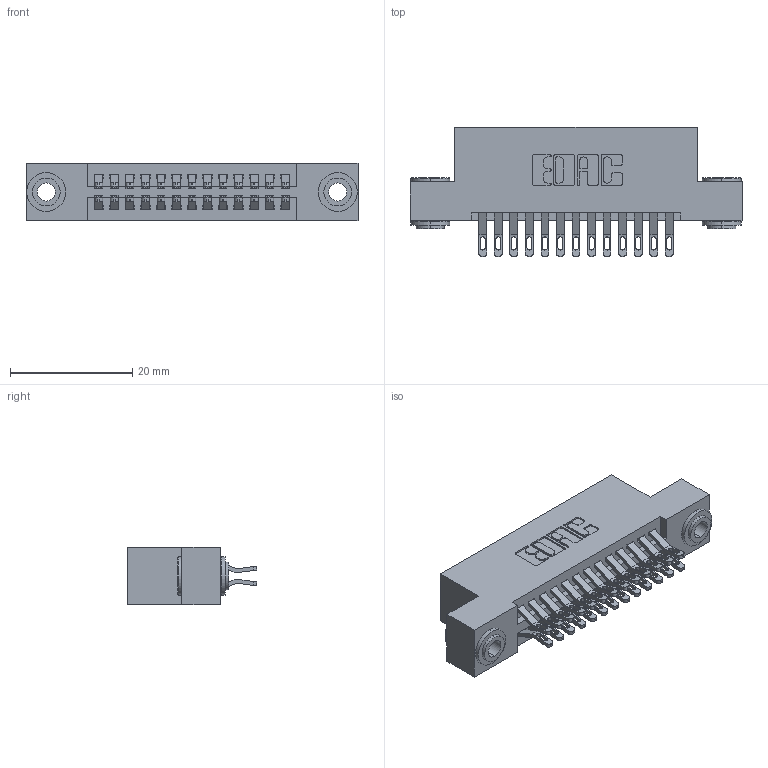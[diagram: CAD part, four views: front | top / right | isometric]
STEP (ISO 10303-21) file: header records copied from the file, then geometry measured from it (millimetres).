
FILE_DESCRIPTION (( 'STEP AP203' ), '1' );
FILE_NAME ('345-026-555-203.STEP', '2019-10-27T19:46:31', ( '' ), ( '' ), 'SwSTEP 2.0', 'SolidWorks 2016', '' );
FILE_SCHEMA (( 'CONFIG_CONTROL_DESIGN' ));
Length unit declared in the file: inch
Products named in the file (4): 345-250-002_345-250-002-102; 345-292-001_555 Tail; 345 Part_Flush Mounting Lugs - 0.156 Dia-TH; 345-026-555-203
Assembly tree (29 placements, depth 2):
  345-026-555-203
    345 Part_Flush Mounting Lugs - 0.156 Dia-TH
    345-292-001_555 Tail  x26
    345-250-002_345-250-002-102  x2
Bounding box: 54.23 x 21.13 x 9.4 mm (x, y, z)
Volume: 5093.5 mm3; surface area: 7434.5 mm2
Topology: 29 solids, 29 shells, 1620 faces, 5019 edges, 3342 vertices
Faces by surface type: plane 896, cylinder 716, cone 8
Entity records: 15080 total; most frequent: CARTESIAN_POINT 2565, ORIENTED_EDGE 2462, DIRECTION 2297, EDGE_CURVE 1231, VECTOR 1003, LINE 1003, VERTEX_POINT 818, AXIS2_PLACEMENT_3D 647
